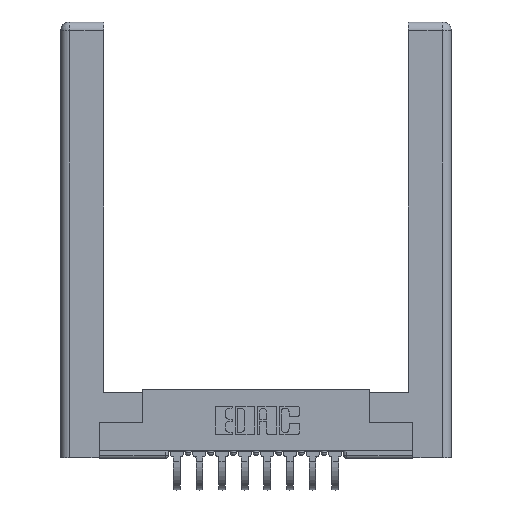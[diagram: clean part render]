
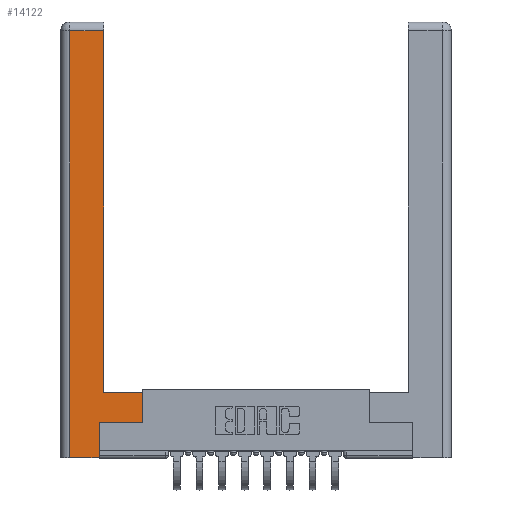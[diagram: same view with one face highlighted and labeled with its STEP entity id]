
A CAD part, top view. The second image highlights one B-rep face of the part: STEP entity #14122.
In plain terms, the highlighted planar face has unit normal (0, 0, 1).
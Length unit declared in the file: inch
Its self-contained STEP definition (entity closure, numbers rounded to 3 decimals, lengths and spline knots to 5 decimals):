
#40 = CARTESIAN_POINT ( 'NONE',  ( 0.565, 0.45, 0. ) ) ;
#197 = FACE_OUTER_BOUND ( 'NONE', #5833, .T. ) ;
#261 = EDGE_CURVE ( 'NONE', #15084, #11873, #705, .T. ) ;
#365 = CARTESIAN_POINT ( 'NONE',  ( 0.565, 0.245, 0. ) ) ;
#467 = ORIENTED_EDGE ( 'NONE', *, *, #9017, .T. ) ;
#705 = LINE ( 'NONE', #15050, #7904 ) ;
#727 = ORIENTED_EDGE ( 'NONE', *, *, #12164, .T. ) ;
#854 = VERTEX_POINT ( 'NONE', #3927 ) ;
#1112 = EDGE_CURVE ( 'NONE', #12796, #13665, #5647, .T. ) ;
#1211 = CARTESIAN_POINT ( 'NONE',  ( 0.565, 0.245, 0. ) ) ;
#1220 = CARTESIAN_POINT ( 'NONE',  ( 0.0615, 2.94, 0. ) ) ;
#1294 = VECTOR ( 'NONE', #7997, 39.37008 ) ;
#1467 = DIRECTION ( 'NONE',  ( 0., -1., 0. ) ) ;
#1690 = DIRECTION ( 'NONE',  ( -1., 0., 0. ) ) ;
#1772 = ORIENTED_EDGE ( 'NONE', *, *, #3644, .T. ) ;
#1852 = CARTESIAN_POINT ( 'NONE',  ( 0., 0., 0. ) ) ;
#2232 = LINE ( 'NONE', #40, #1294 ) ;
#2337 = DIRECTION ( 'NONE',  ( 1., 0., 0. ) ) ;
#3449 = EDGE_CURVE ( 'NONE', #13665, #14554, #4038, .T. ) ;
#3644 = EDGE_CURVE ( 'NONE', #14554, #15084, #2232, .T. ) ;
#3888 = LINE ( 'NONE', #14325, #13256 ) ;
#3927 = CARTESIAN_POINT ( 'NONE',  ( 0.0615, 2.94, 0. ) ) ;
#4038 = LINE ( 'NONE', #365, #8263 ) ;
#4281 = CARTESIAN_POINT ( 'NONE',  ( 0.565, 0.45, 0. ) ) ;
#4398 = DIRECTION ( 'NONE',  ( 0., 1., 0. ) ) ;
#4699 = EDGE_CURVE ( 'NONE', #11873, #12456, #9822, .T. ) ;
#5079 = CARTESIAN_POINT ( 'NONE',  ( 0.295, 0.45, 0. ) ) ;
#5265 = AXIS2_PLACEMENT_3D ( 'NONE', #1852, #6604, #1690 ) ;
#5647 = LINE ( 'NONE', #15144, #12718 ) ;
#5833 = EDGE_LOOP ( 'NONE', ( #7909, #467, #12232, #727, #12030, #11138, #1772, #9279 ) ) ;
#6049 = DIRECTION ( 'NONE',  ( -1., 0., 0. ) ) ;
#6604 = DIRECTION ( 'NONE',  ( 0., 0., -1. ) ) ;
#7399 = CARTESIAN_POINT ( 'NONE',  ( 0.295, 3., 0. ) ) ;
#7608 = CARTESIAN_POINT ( 'NONE',  ( 0.0615, 0., 0. ) ) ;
#7625 = CARTESIAN_POINT ( 'NONE',  ( 0.295, 2.94, 0. ) ) ;
#7904 = VECTOR ( 'NONE', #7943, 39.37008 ) ;
#7909 = ORIENTED_EDGE ( 'NONE', *, *, #4699, .T. ) ;
#7943 = DIRECTION ( 'NONE',  ( -1., 0., 0. ) ) ;
#7997 = DIRECTION ( 'NONE',  ( 0., 1., 0. ) ) ;
#8263 = VECTOR ( 'NONE', #8792, 39.37008 ) ;
#8266 = DIRECTION ( 'NONE',  ( 0., 1., 0. ) ) ;
#8552 = EDGE_CURVE ( 'NONE', #854, #9163, #3888, .T. ) ;
#8792 = DIRECTION ( 'NONE',  ( 1., 0., 0. ) ) ;
#9017 = EDGE_CURVE ( 'NONE', #12456, #854, #11033, .T. ) ;
#9163 = VERTEX_POINT ( 'NONE', #7608 ) ;
#9188 = CARTESIAN_POINT ( 'NONE',  ( 0.265, 0.245, 0. ) ) ;
#9279 = ORIENTED_EDGE ( 'NONE', *, *, #261, .T. ) ;
#9712 = PLANE ( 'NONE',  #5265 ) ;
#9822 = LINE ( 'NONE', #7399, #12586 ) ;
#10062 = VECTOR ( 'NONE', #6049, 39.37008 ) ;
#11033 = LINE ( 'NONE', #1220, #10062 ) ;
#11138 = ORIENTED_EDGE ( 'NONE', *, *, #3449, .T. ) ;
#11873 = VERTEX_POINT ( 'NONE', #5079 ) ;
#12030 = ORIENTED_EDGE ( 'NONE', *, *, #1112, .T. ) ;
#12071 = VECTOR ( 'NONE', #2337, 39.37008 ) ;
#12164 = EDGE_CURVE ( 'NONE', #9163, #12796, #14025, .T. ) ;
#12232 = ORIENTED_EDGE ( 'NONE', *, *, #8552, .T. ) ;
#12456 = VERTEX_POINT ( 'NONE', #7625 ) ;
#12586 = VECTOR ( 'NONE', #8266, 39.37008 ) ;
#12718 = VECTOR ( 'NONE', #4398, 39.37008 ) ;
#12796 = VERTEX_POINT ( 'NONE', #13586 ) ;
#13256 = VECTOR ( 'NONE', #1467, 39.37008 ) ;
#13586 = CARTESIAN_POINT ( 'NONE',  ( 0.265, 0., 0. ) ) ;
#13665 = VERTEX_POINT ( 'NONE', #9188 ) ;
#14025 = LINE ( 'NONE', #15199, #12071 ) ;
#14122 = ADVANCED_FACE ( 'NONE', ( #197 ), #9712, .F. ) ;
#14325 = CARTESIAN_POINT ( 'NONE',  ( 0.0615, 0., 0. ) ) ;
#14554 = VERTEX_POINT ( 'NONE', #1211 ) ;
#15050 = CARTESIAN_POINT ( 'NONE',  ( 0.295, 0.45, 0. ) ) ;
#15084 = VERTEX_POINT ( 'NONE', #4281 ) ;
#15144 = CARTESIAN_POINT ( 'NONE',  ( 0.265, 0.245, 0. ) ) ;
#15199 = CARTESIAN_POINT ( 'NONE',  ( 0.265, 0., 0. ) ) ;
